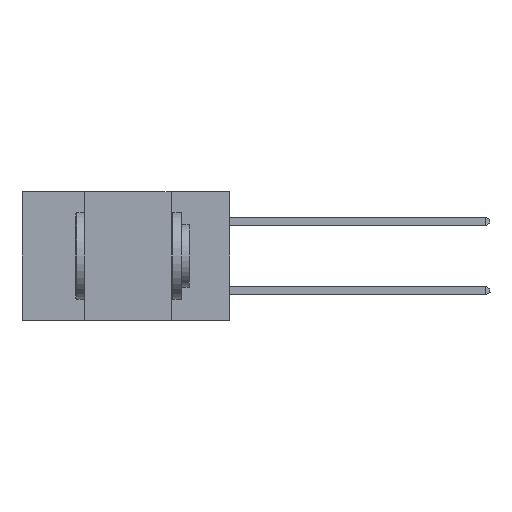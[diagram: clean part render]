
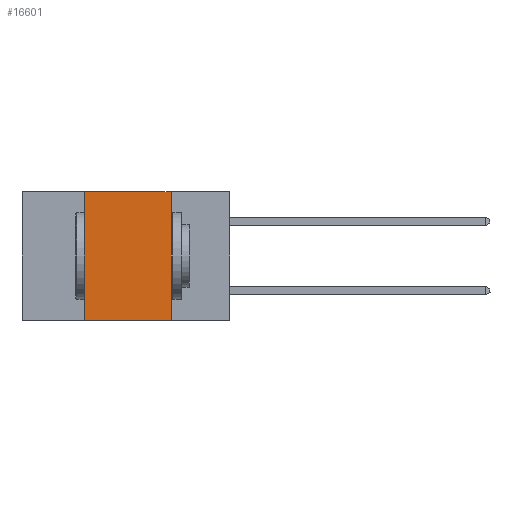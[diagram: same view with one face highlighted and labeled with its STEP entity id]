
A CAD part, left-side view. The second image highlights one B-rep face of the part: STEP entity #16601.
In plain terms, the highlighted planar face has unit normal (-1, 0, 0).
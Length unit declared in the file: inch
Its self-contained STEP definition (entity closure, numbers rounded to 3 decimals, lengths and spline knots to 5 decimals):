
#986 = VECTOR ( 'NONE', #8232, 39.37008 ) ;
#1556 = ORIENTED_EDGE ( 'NONE', *, *, #12420, .F. ) ;
#2814 = CARTESIAN_POINT ( 'NONE',  ( 0., 0.6, -0.37 ) ) ;
#2861 = AXIS2_PLACEMENT_3D ( 'NONE', #18605, #24565, #22489 ) ;
#3306 = FACE_OUTER_BOUND ( 'NONE', #12389, .T. ) ;
#3383 = CARTESIAN_POINT ( 'NONE',  ( 0., 0.42, 0. ) ) ;
#3521 = VERTEX_POINT ( 'NONE', #8440 ) ;
#4984 = PLANE ( 'NONE',  #2861 ) ;
#5881 = LINE ( 'NONE', #2814, #20393 ) ;
#6392 = CARTESIAN_POINT ( 'NONE',  ( 0., 0.6, 0. ) ) ;
#6619 = ORIENTED_EDGE ( 'NONE', *, *, #7742, .F. ) ;
#7742 = EDGE_CURVE ( 'NONE', #13633, #8518, #9377, .T. ) ;
#8232 = DIRECTION ( 'NONE',  ( 0., 0., 1. ) ) ;
#8440 = CARTESIAN_POINT ( 'NONE',  ( 0., 0.17, 0. ) ) ;
#8518 = VERTEX_POINT ( 'NONE', #3383 ) ;
#9377 = LINE ( 'NONE', #12530, #986 ) ;
#9572 = CARTESIAN_POINT ( 'NONE',  ( 0., 0.17, -0.37 ) ) ;
#10243 = ORIENTED_EDGE ( 'NONE', *, *, #10422, .T. ) ;
#10422 = EDGE_CURVE ( 'NONE', #13633, #25486, #5881, .T. ) ;
#11045 = LINE ( 'NONE', #6392, #23103 ) ;
#11837 = EDGE_CURVE ( 'NONE', #8518, #3521, #11045, .T. ) ;
#12252 = DIRECTION ( 'NONE',  ( 0., -1., 0. ) ) ;
#12389 = EDGE_LOOP ( 'NONE', ( #1556, #18398, #6619, #10243 ) ) ;
#12420 = EDGE_CURVE ( 'NONE', #3521, #25486, #15591, .T. ) ;
#12530 = CARTESIAN_POINT ( 'NONE',  ( 0., 0.42, 0. ) ) ;
#13633 = VERTEX_POINT ( 'NONE', #23069 ) ;
#15591 = LINE ( 'NONE', #21900, #19337 ) ;
#16601 = ADVANCED_FACE ( 'NONE', ( #3306 ), #4984, .F. ) ;
#18398 = ORIENTED_EDGE ( 'NONE', *, *, #11837, .F. ) ;
#18605 = CARTESIAN_POINT ( 'NONE',  ( 0., 0.6, 0. ) ) ;
#19337 = VECTOR ( 'NONE', #21718, 39.37008 ) ;
#20393 = VECTOR ( 'NONE', #20642, 39.37008 ) ;
#20642 = DIRECTION ( 'NONE',  ( 0., -1., 0. ) ) ;
#21718 = DIRECTION ( 'NONE',  ( 0., 0., -1. ) ) ;
#21900 = CARTESIAN_POINT ( 'NONE',  ( 0., 0.17, 0. ) ) ;
#22489 = DIRECTION ( 'NONE',  ( 0., 0., -1. ) ) ;
#23069 = CARTESIAN_POINT ( 'NONE',  ( 0., 0.42, -0.37 ) ) ;
#23103 = VECTOR ( 'NONE', #12252, 39.37008 ) ;
#24565 = DIRECTION ( 'NONE',  ( 1., 0., 0. ) ) ;
#25486 = VERTEX_POINT ( 'NONE', #9572 ) ;
